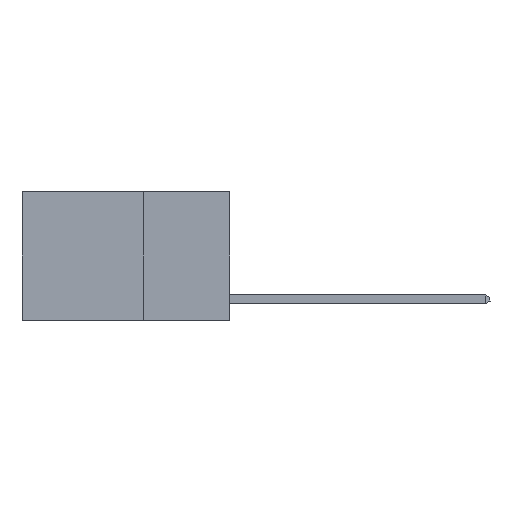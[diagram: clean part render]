
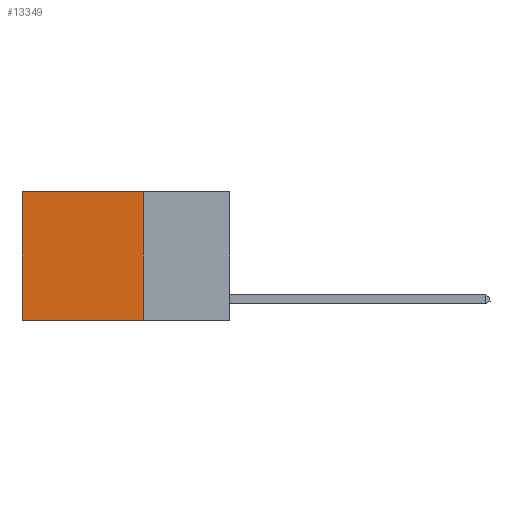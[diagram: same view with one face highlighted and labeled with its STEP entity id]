
A CAD part, left-side view. The second image highlights one B-rep face of the part: STEP entity #13349.
In plain terms, the highlighted planar face has unit normal (-1, 0, 0).
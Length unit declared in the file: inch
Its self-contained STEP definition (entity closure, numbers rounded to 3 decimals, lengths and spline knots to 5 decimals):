
#455 = ORIENTED_EDGE ( 'NONE', *, *, #5691, .T. ) ;
#531 = EDGE_CURVE ( 'NONE', #14834, #4515, #15049, .T. ) ;
#1012 = LINE ( 'NONE', #19678, #21927 ) ;
#1227 = VECTOR ( 'NONE', #20756, 39.37008 ) ;
#2204 = ORIENTED_EDGE ( 'NONE', *, *, #8092, .T. ) ;
#3342 = FACE_OUTER_BOUND ( 'NONE', #11390, .T. ) ;
#4515 = VERTEX_POINT ( 'NONE', #16026 ) ;
#5324 = AXIS2_PLACEMENT_3D ( 'NONE', #15346, #11964, #17539 ) ;
#5691 = EDGE_CURVE ( 'NONE', #14834, #18000, #5906, .T. ) ;
#5756 = LINE ( 'NONE', #7109, #1227 ) ;
#5906 = LINE ( 'NONE', #20402, #18874 ) ;
#7109 = CARTESIAN_POINT ( 'NONE',  ( 0.2625, 0.25, -0.37 ) ) ;
#7414 = ORIENTED_EDGE ( 'NONE', *, *, #21152, .F. ) ;
#8092 = EDGE_CURVE ( 'NONE', #18000, #8676, #1012, .T. ) ;
#8676 = VERTEX_POINT ( 'NONE', #9616 ) ;
#8990 = CARTESIAN_POINT ( 'NONE',  ( 0.2625, 0.25, 0. ) ) ;
#9518 = CARTESIAN_POINT ( 'NONE',  ( 0.2625, 0.25, 0. ) ) ;
#9616 = CARTESIAN_POINT ( 'NONE',  ( 0.2625, 0.6, -0.37 ) ) ;
#9924 = DIRECTION ( 'NONE',  ( 0., 0., -1. ) ) ;
#11390 = EDGE_LOOP ( 'NONE', ( #2204, #7414, #14156, #455 ) ) ;
#11964 = DIRECTION ( 'NONE',  ( 1., 0., 0. ) ) ;
#12036 = DIRECTION ( 'NONE',  ( 0., 1., 0. ) ) ;
#12212 = CARTESIAN_POINT ( 'NONE',  ( 0.2625, 0.6, 0. ) ) ;
#12406 = VECTOR ( 'NONE', #21202, 39.37008 ) ;
#13349 = ADVANCED_FACE ( 'NONE', ( #3342 ), #21399, .F. ) ;
#14156 = ORIENTED_EDGE ( 'NONE', *, *, #531, .F. ) ;
#14834 = VERTEX_POINT ( 'NONE', #8990 ) ;
#15049 = LINE ( 'NONE', #9518, #12406 ) ;
#15346 = CARTESIAN_POINT ( 'NONE',  ( 0.2625, 0.25, 0. ) ) ;
#16026 = CARTESIAN_POINT ( 'NONE',  ( 0.2625, 0.25, -0.37 ) ) ;
#17539 = DIRECTION ( 'NONE',  ( 0., 0., -1. ) ) ;
#18000 = VERTEX_POINT ( 'NONE', #12212 ) ;
#18874 = VECTOR ( 'NONE', #12036, 39.37008 ) ;
#19678 = CARTESIAN_POINT ( 'NONE',  ( 0.2625, 0.6, 0. ) ) ;
#20402 = CARTESIAN_POINT ( 'NONE',  ( 0.2625, 0.25, 0. ) ) ;
#20756 = DIRECTION ( 'NONE',  ( 0., 1., 0. ) ) ;
#21152 = EDGE_CURVE ( 'NONE', #4515, #8676, #5756, .T. ) ;
#21202 = DIRECTION ( 'NONE',  ( 0., 0., -1. ) ) ;
#21399 = PLANE ( 'NONE',  #5324 ) ;
#21927 = VECTOR ( 'NONE', #9924, 39.37008 ) ;
